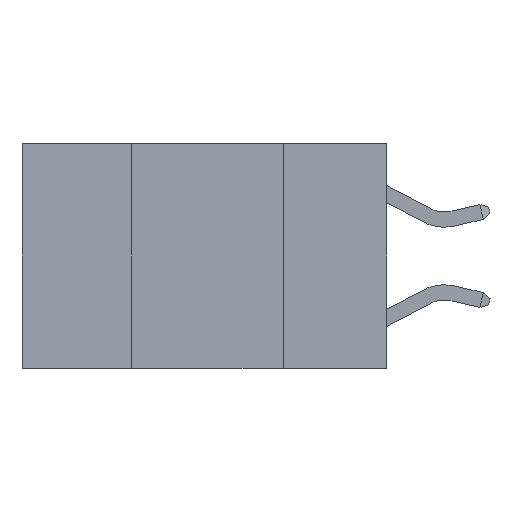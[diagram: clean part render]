
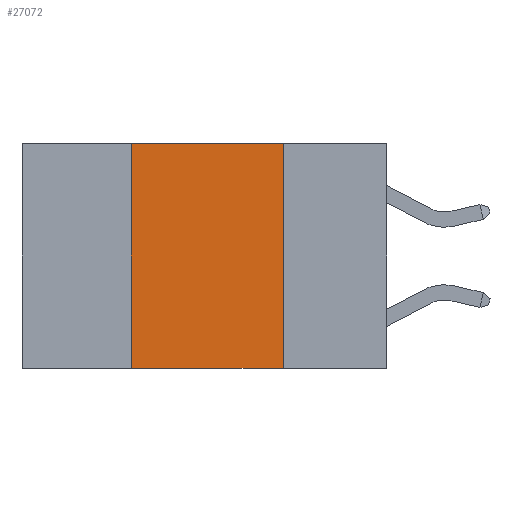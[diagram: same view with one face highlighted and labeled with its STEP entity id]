
A CAD part, left-side view. The second image highlights one B-rep face of the part: STEP entity #27072.
In plain terms, the highlighted planar face has unit normal (-1, 0, 0).
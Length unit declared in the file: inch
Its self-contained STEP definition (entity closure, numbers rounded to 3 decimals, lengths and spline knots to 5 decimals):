
#414 = CARTESIAN_POINT ( 'NONE',  ( 0., 0.6, 0. ) ) ;
#1587 = DIRECTION ( 'NONE',  ( 0., -1., 0. ) ) ;
#1660 = ORIENTED_EDGE ( 'NONE', *, *, #27319, .F. ) ;
#1733 = LINE ( 'NONE', #26473, #17226 ) ;
#2236 = CARTESIAN_POINT ( 'NONE',  ( 0., 0.6, -0.37 ) ) ;
#3357 = LINE ( 'NONE', #414, #4515 ) ;
#3679 = DIRECTION ( 'NONE',  ( 0., -1., 0. ) ) ;
#4515 = VECTOR ( 'NONE', #3679, 39.37008 ) ;
#5134 = CARTESIAN_POINT ( 'NONE',  ( 0., 0.17, 0. ) ) ;
#6570 = VECTOR ( 'NONE', #1587, 39.37008 ) ;
#6738 = EDGE_CURVE ( 'NONE', #7186, #14286, #3357, .T. ) ;
#6879 = PLANE ( 'NONE',  #12017 ) ;
#7186 = VERTEX_POINT ( 'NONE', #23384 ) ;
#8567 = VERTEX_POINT ( 'NONE', #28614 ) ;
#9639 = DIRECTION ( 'NONE',  ( 0., 0., -1. ) ) ;
#11450 = CARTESIAN_POINT ( 'NONE',  ( 0., 0.6, 0. ) ) ;
#11502 = VECTOR ( 'NONE', #24903, 39.37008 ) ;
#11698 = DIRECTION ( 'NONE',  ( 0., 0., -1. ) ) ;
#12017 = AXIS2_PLACEMENT_3D ( 'NONE', #11450, #31954, #9639 ) ;
#12184 = ORIENTED_EDGE ( 'NONE', *, *, #19966, .T. ) ;
#14286 = VERTEX_POINT ( 'NONE', #5134 ) ;
#14893 = CARTESIAN_POINT ( 'NONE',  ( 0., 0.42, 0. ) ) ;
#17163 = LINE ( 'NONE', #2236, #6570 ) ;
#17226 = VECTOR ( 'NONE', #11698, 39.37008 ) ;
#18660 = ORIENTED_EDGE ( 'NONE', *, *, #28096, .F. ) ;
#19966 = EDGE_CURVE ( 'NONE', #8567, #24529, #17163, .T. ) ;
#23384 = CARTESIAN_POINT ( 'NONE',  ( 0., 0.42, 0. ) ) ;
#24491 = EDGE_LOOP ( 'NONE', ( #18660, #24547, #1660, #12184 ) ) ;
#24529 = VERTEX_POINT ( 'NONE', #27511 ) ;
#24547 = ORIENTED_EDGE ( 'NONE', *, *, #6738, .F. ) ;
#24903 = DIRECTION ( 'NONE',  ( 0., 0., 1. ) ) ;
#26473 = CARTESIAN_POINT ( 'NONE',  ( 0., 0.17, 0. ) ) ;
#27072 = ADVANCED_FACE ( 'NONE', ( #29485 ), #6879, .F. ) ;
#27319 = EDGE_CURVE ( 'NONE', #8567, #7186, #27364, .T. ) ;
#27364 = LINE ( 'NONE', #14893, #11502 ) ;
#27511 = CARTESIAN_POINT ( 'NONE',  ( 0., 0.17, -0.37 ) ) ;
#28096 = EDGE_CURVE ( 'NONE', #14286, #24529, #1733, .T. ) ;
#28614 = CARTESIAN_POINT ( 'NONE',  ( 0., 0.42, -0.37 ) ) ;
#29485 = FACE_OUTER_BOUND ( 'NONE', #24491, .T. ) ;
#31954 = DIRECTION ( 'NONE',  ( 1., 0., 0. ) ) ;
